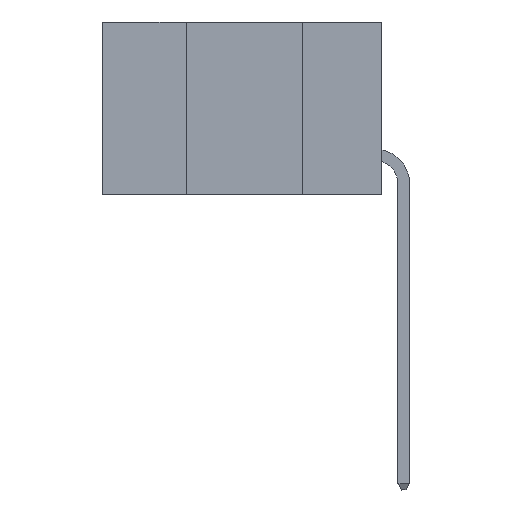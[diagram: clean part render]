
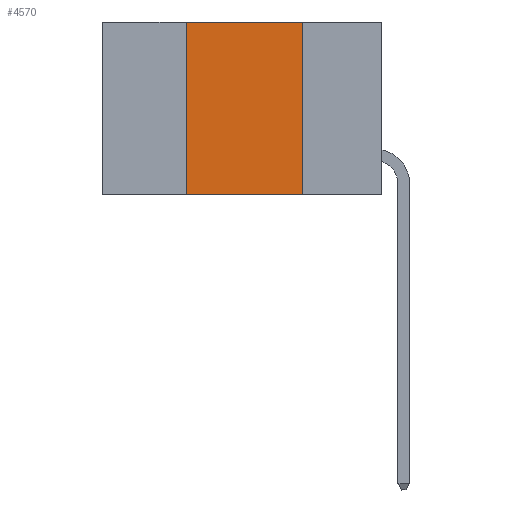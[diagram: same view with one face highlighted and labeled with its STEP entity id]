
A CAD part, left-side view. The second image highlights one B-rep face of the part: STEP entity #4570.
In plain terms, the highlighted planar face has unit normal (-1, 0, 0).
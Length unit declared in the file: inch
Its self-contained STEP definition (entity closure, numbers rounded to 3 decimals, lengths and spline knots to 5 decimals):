
#1064 = VERTEX_POINT ( 'NONE', #6655 ) ;
#1142 = CARTESIAN_POINT ( 'NONE',  ( 0., 0.6, 0. ) ) ;
#1717 = LINE ( 'NONE', #2317, #19829 ) ;
#1806 = DIRECTION ( 'NONE',  ( 0., 0., -1. ) ) ;
#1862 = LINE ( 'NONE', #16787, #12981 ) ;
#2301 = ORIENTED_EDGE ( 'NONE', *, *, #12840, .F. ) ;
#2317 = CARTESIAN_POINT ( 'NONE',  ( 0., 0.17, 0. ) ) ;
#3153 = VECTOR ( 'NONE', #17609, 39.37008 ) ;
#3825 = VERTEX_POINT ( 'NONE', #17197 ) ;
#4570 = ADVANCED_FACE ( 'NONE', ( #18428 ), #13550, .F. ) ;
#5380 = ORIENTED_EDGE ( 'NONE', *, *, #11952, .F. ) ;
#5428 = VERTEX_POINT ( 'NONE', #17163 ) ;
#6655 = CARTESIAN_POINT ( 'NONE',  ( 0., 0.17, -0.37 ) ) ;
#6841 = CARTESIAN_POINT ( 'NONE',  ( 0., 0.42, 0. ) ) ;
#7573 = VECTOR ( 'NONE', #10550, 39.37008 ) ;
#8817 = CARTESIAN_POINT ( 'NONE',  ( 0., 0.17, 0. ) ) ;
#8931 = CARTESIAN_POINT ( 'NONE',  ( 0., 0.6, 0. ) ) ;
#9809 = ORIENTED_EDGE ( 'NONE', *, *, #12532, .F. ) ;
#10550 = DIRECTION ( 'NONE',  ( 0., -1., 0. ) ) ;
#11356 = AXIS2_PLACEMENT_3D ( 'NONE', #8931, #15000, #16343 ) ;
#11952 = EDGE_CURVE ( 'NONE', #3825, #13165, #12149, .T. ) ;
#12149 = LINE ( 'NONE', #1142, #7573 ) ;
#12532 = EDGE_CURVE ( 'NONE', #13165, #1064, #1717, .T. ) ;
#12840 = EDGE_CURVE ( 'NONE', #5428, #3825, #20050, .T. ) ;
#12981 = VECTOR ( 'NONE', #20011, 39.37008 ) ;
#13165 = VERTEX_POINT ( 'NONE', #8817 ) ;
#13550 = PLANE ( 'NONE',  #11356 ) ;
#14868 = EDGE_CURVE ( 'NONE', #5428, #1064, #1862, .T. ) ;
#15000 = DIRECTION ( 'NONE',  ( 1., 0., 0. ) ) ;
#16343 = DIRECTION ( 'NONE',  ( 0., 0., -1. ) ) ;
#16787 = CARTESIAN_POINT ( 'NONE',  ( 0., 0.6, -0.37 ) ) ;
#17163 = CARTESIAN_POINT ( 'NONE',  ( 0., 0.42, -0.37 ) ) ;
#17197 = CARTESIAN_POINT ( 'NONE',  ( 0., 0.42, 0. ) ) ;
#17609 = DIRECTION ( 'NONE',  ( 0., 0., 1. ) ) ;
#18260 = ORIENTED_EDGE ( 'NONE', *, *, #14868, .T. ) ;
#18428 = FACE_OUTER_BOUND ( 'NONE', #18755, .T. ) ;
#18755 = EDGE_LOOP ( 'NONE', ( #9809, #5380, #2301, #18260 ) ) ;
#19829 = VECTOR ( 'NONE', #1806, 39.37008 ) ;
#20011 = DIRECTION ( 'NONE',  ( 0., -1., 0. ) ) ;
#20050 = LINE ( 'NONE', #6841, #3153 ) ;
